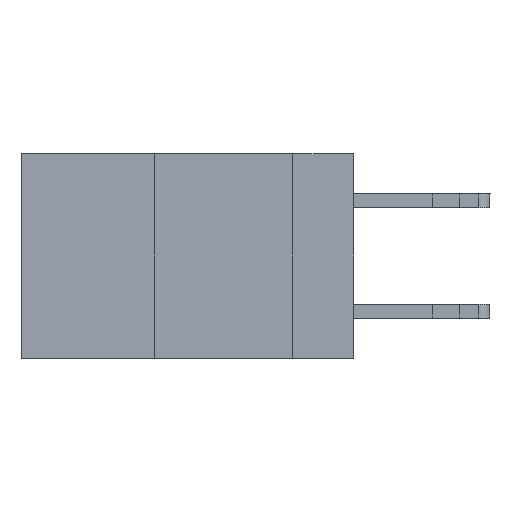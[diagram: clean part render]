
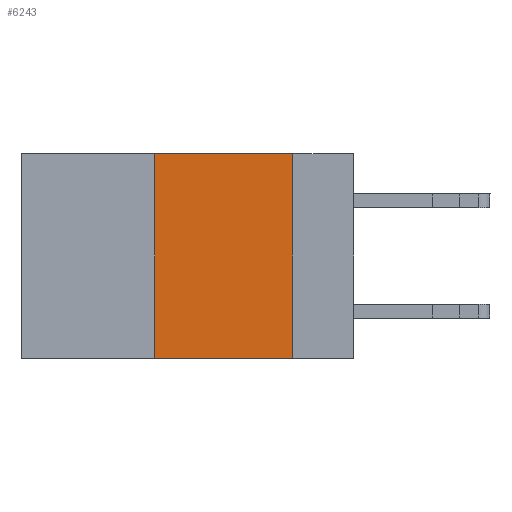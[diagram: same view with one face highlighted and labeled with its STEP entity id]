
A CAD part, left-side view. The second image highlights one B-rep face of the part: STEP entity #6243.
In plain terms, the highlighted planar face has unit normal (-1, 0, 0).
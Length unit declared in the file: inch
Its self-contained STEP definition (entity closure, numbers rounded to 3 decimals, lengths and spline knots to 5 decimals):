
#235 = ORIENTED_EDGE ( 'NONE', *, *, #10422, .T. ) ;
#749 = CARTESIAN_POINT ( 'NONE',  ( 0., 0.36, 0. ) ) ;
#1137 = VERTEX_POINT ( 'NONE', #749 ) ;
#1409 = LINE ( 'NONE', #12075, #6029 ) ;
#1518 = VERTEX_POINT ( 'NONE', #3646 ) ;
#2497 = EDGE_CURVE ( 'NONE', #1137, #1518, #10305, .T. ) ;
#2520 = CARTESIAN_POINT ( 'NONE',  ( 0., 0.11, 0. ) ) ;
#3646 = CARTESIAN_POINT ( 'NONE',  ( 0., 0.11, 0. ) ) ;
#3655 = ORIENTED_EDGE ( 'NONE', *, *, #15015, .F. ) ;
#3691 = DIRECTION ( 'NONE',  ( 0., 0., 1. ) ) ;
#4115 = LINE ( 'NONE', #7813, #7896 ) ;
#4309 = VECTOR ( 'NONE', #14771, 39.37008 ) ;
#5058 = ORIENTED_EDGE ( 'NONE', *, *, #2497, .F. ) ;
#5962 = EDGE_LOOP ( 'NONE', ( #9879, #5058, #3655, #235 ) ) ;
#6029 = VECTOR ( 'NONE', #3691, 39.37008 ) ;
#6115 = VECTOR ( 'NONE', #16620, 39.37008 ) ;
#6243 = ADVANCED_FACE ( 'NONE', ( #11674 ), #6836, .F. ) ;
#6401 = DIRECTION ( 'NONE',  ( 0., -1., 0. ) ) ;
#6836 = PLANE ( 'NONE',  #9218 ) ;
#7813 = CARTESIAN_POINT ( 'NONE',  ( 0., 0.6, -0.37 ) ) ;
#7896 = VECTOR ( 'NONE', #6401, 39.37008 ) ;
#9218 = AXIS2_PLACEMENT_3D ( 'NONE', #16299, #9532, #9642 ) ;
#9532 = DIRECTION ( 'NONE',  ( 1., 0., 0. ) ) ;
#9642 = DIRECTION ( 'NONE',  ( 0., 0., -1. ) ) ;
#9879 = ORIENTED_EDGE ( 'NONE', *, *, #15583, .F. ) ;
#10305 = LINE ( 'NONE', #12540, #6115 ) ;
#10422 = EDGE_CURVE ( 'NONE', #15078, #14265, #4115, .T. ) ;
#11674 = FACE_OUTER_BOUND ( 'NONE', #5962, .T. ) ;
#11821 = CARTESIAN_POINT ( 'NONE',  ( 0., 0.36, -0.37 ) ) ;
#12075 = CARTESIAN_POINT ( 'NONE',  ( 0., 0.36, 0. ) ) ;
#12540 = CARTESIAN_POINT ( 'NONE',  ( 0., 0.6, 0. ) ) ;
#14265 = VERTEX_POINT ( 'NONE', #15119 ) ;
#14771 = DIRECTION ( 'NONE',  ( 0., 0., -1. ) ) ;
#15015 = EDGE_CURVE ( 'NONE', #15078, #1137, #1409, .T. ) ;
#15078 = VERTEX_POINT ( 'NONE', #11821 ) ;
#15119 = CARTESIAN_POINT ( 'NONE',  ( 0., 0.11, -0.37 ) ) ;
#15525 = LINE ( 'NONE', #2520, #4309 ) ;
#15583 = EDGE_CURVE ( 'NONE', #1518, #14265, #15525, .T. ) ;
#16299 = CARTESIAN_POINT ( 'NONE',  ( 0., 0.6, 0. ) ) ;
#16620 = DIRECTION ( 'NONE',  ( 0., -1., 0. ) ) ;
